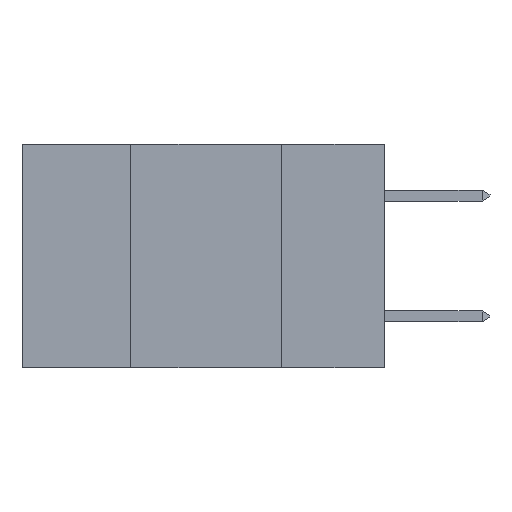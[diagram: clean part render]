
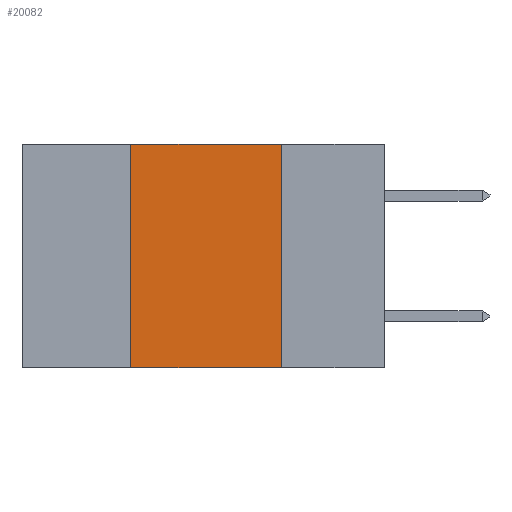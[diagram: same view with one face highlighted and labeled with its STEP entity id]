
A CAD part, left-side view. The second image highlights one B-rep face of the part: STEP entity #20082.
In plain terms, the highlighted planar face has unit normal (-1, 0, 0).
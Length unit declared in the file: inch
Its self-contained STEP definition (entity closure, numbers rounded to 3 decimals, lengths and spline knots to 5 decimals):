
#132 = CARTESIAN_POINT ( 'NONE',  ( 0., 0.6, 0. ) ) ;
#241 = VERTEX_POINT ( 'NONE', #7821 ) ;
#1265 = LINE ( 'NONE', #5512, #11165 ) ;
#2067 = VERTEX_POINT ( 'NONE', #19620 ) ;
#2105 = DIRECTION ( 'NONE',  ( 0., 0., -1. ) ) ;
#3985 = PLANE ( 'NONE',  #23458 ) ;
#4097 = VECTOR ( 'NONE', #4185, 39.37008 ) ;
#4185 = DIRECTION ( 'NONE',  ( 0., 0., 1. ) ) ;
#4263 = CARTESIAN_POINT ( 'NONE',  ( 0., 0.42, 0. ) ) ;
#4740 = VECTOR ( 'NONE', #18960, 39.37008 ) ;
#5512 = CARTESIAN_POINT ( 'NONE',  ( 0., 0.6, -0.37 ) ) ;
#6515 = CARTESIAN_POINT ( 'NONE',  ( 0., 0.42, -0.37 ) ) ;
#6538 = VERTEX_POINT ( 'NONE', #23690 ) ;
#7524 = DIRECTION ( 'NONE',  ( 0., -1., 0. ) ) ;
#7821 = CARTESIAN_POINT ( 'NONE',  ( 0., 0.17, -0.37 ) ) ;
#10129 = EDGE_CURVE ( 'NONE', #13974, #2067, #16709, .T. ) ;
#11165 = VECTOR ( 'NONE', #7524, 39.37008 ) ;
#12073 = LINE ( 'NONE', #12859, #22285 ) ;
#12429 = ORIENTED_EDGE ( 'NONE', *, *, #25111, .F. ) ;
#12859 = CARTESIAN_POINT ( 'NONE',  ( 0., 0.17, 0. ) ) ;
#13453 = EDGE_LOOP ( 'NONE', ( #12429, #20427, #16291, #19490 ) ) ;
#13974 = VERTEX_POINT ( 'NONE', #6515 ) ;
#14033 = DIRECTION ( 'NONE',  ( 1., 0., 0. ) ) ;
#14914 = DIRECTION ( 'NONE',  ( 0., 0., -1. ) ) ;
#16291 = ORIENTED_EDGE ( 'NONE', *, *, #10129, .F. ) ;
#16709 = LINE ( 'NONE', #4263, #4097 ) ;
#16914 = CARTESIAN_POINT ( 'NONE',  ( 0., 0.6, 0. ) ) ;
#17851 = EDGE_CURVE ( 'NONE', #13974, #241, #1265, .T. ) ;
#18960 = DIRECTION ( 'NONE',  ( 0., -1., 0. ) ) ;
#19490 = ORIENTED_EDGE ( 'NONE', *, *, #17851, .T. ) ;
#19620 = CARTESIAN_POINT ( 'NONE',  ( 0., 0.42, 0. ) ) ;
#19765 = FACE_OUTER_BOUND ( 'NONE', #13453, .T. ) ;
#20082 = ADVANCED_FACE ( 'NONE', ( #19765 ), #3985, .F. ) ;
#20427 = ORIENTED_EDGE ( 'NONE', *, *, #23007, .F. ) ;
#20864 = LINE ( 'NONE', #16914, #4740 ) ;
#22285 = VECTOR ( 'NONE', #14914, 39.37008 ) ;
#23007 = EDGE_CURVE ( 'NONE', #2067, #6538, #20864, .T. ) ;
#23458 = AXIS2_PLACEMENT_3D ( 'NONE', #132, #14033, #2105 ) ;
#23690 = CARTESIAN_POINT ( 'NONE',  ( 0., 0.17, 0. ) ) ;
#25111 = EDGE_CURVE ( 'NONE', #6538, #241, #12073, .T. ) ;
